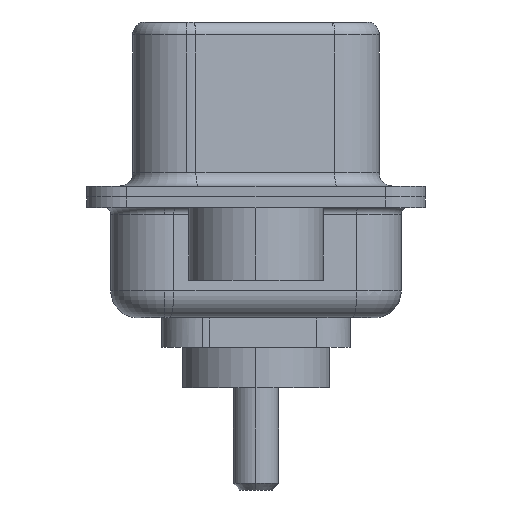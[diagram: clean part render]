
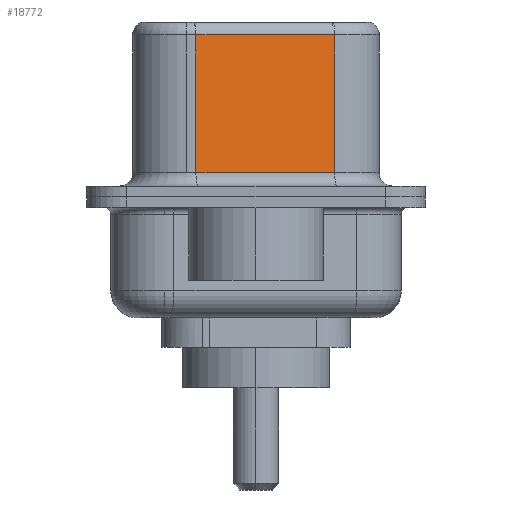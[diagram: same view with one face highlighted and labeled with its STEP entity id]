
A CAD part, left-side view. The second image highlights one B-rep face of the part: STEP entity #18772.
In plain terms, the highlighted planar face has unit normal (-0.985, -0.174, 0).
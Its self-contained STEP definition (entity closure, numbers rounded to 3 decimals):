
#377 = EDGE_LOOP ( 'NONE', ( #16490, #16355, #4769, #13958 ) ) ;
#455 = EDGE_CURVE ( 'NONE', #14845, #7604, #10488, .T. ) ;
#514 = EDGE_CURVE ( 'NONE', #8556, #4223, #520, .T. ) ;
#520 = LINE ( 'NONE', #18550, #5027 ) ;
#2839 = LINE ( 'NONE', #10534, #11919 ) ;
#3498 = DIRECTION ( 'NONE',  ( -0.174, 0.985, 0. ) ) ;
#3651 = CARTESIAN_POINT ( 'NONE',  ( 3.67, 2.233, 6.52 ) ) ;
#3732 = DIRECTION ( 'NONE',  ( 0.985, 0.174, 0. ) ) ;
#4147 = LINE ( 'NONE', #3651, #4860 ) ;
#4223 = VERTEX_POINT ( 'NONE', #9296 ) ;
#4769 = ORIENTED_EDGE ( 'NONE', *, *, #16687, .T. ) ;
#4860 = VECTOR ( 'NONE', #18268, 1000. ) ;
#5027 = VECTOR ( 'NONE', #13930, 1000. ) ;
#5991 = CARTESIAN_POINT ( 'NONE',  ( 4.58, -2.927, 6.02 ) ) ;
#7093 = DIRECTION ( 'NONE',  ( -0.174, 0.985, 0. ) ) ;
#7278 = CARTESIAN_POINT ( 'NONE',  ( 3.67, 2.233, 0.9 ) ) ;
#7604 = VERTEX_POINT ( 'NONE', #16221 ) ;
#8195 = PLANE ( 'NONE',  #8287 ) ;
#8287 = AXIS2_PLACEMENT_3D ( 'NONE', #18180, #3732, #7093 ) ;
#8556 = VERTEX_POINT ( 'NONE', #7278 ) ;
#9296 = CARTESIAN_POINT ( 'NONE',  ( 4.58, -2.927, 0.9 ) ) ;
#9544 = CARTESIAN_POINT ( 'NONE',  ( 4.58, -2.927, 6.02 ) ) ;
#10476 = DIRECTION ( 'NONE',  ( 0., 0., -1. ) ) ;
#10488 = LINE ( 'NONE', #9544, #17499 ) ;
#10534 = CARTESIAN_POINT ( 'NONE',  ( 4.58, -2.927, 6.52 ) ) ;
#11919 = VECTOR ( 'NONE', #10476, 1000. ) ;
#13930 = DIRECTION ( 'NONE',  ( 0.174, -0.985, 0. ) ) ;
#13958 = ORIENTED_EDGE ( 'NONE', *, *, #514, .T. ) ;
#14845 = VERTEX_POINT ( 'NONE', #5991 ) ;
#15698 = EDGE_CURVE ( 'NONE', #14845, #4223, #2839, .T. ) ;
#16221 = CARTESIAN_POINT ( 'NONE',  ( 3.67, 2.233, 6.02 ) ) ;
#16355 = ORIENTED_EDGE ( 'NONE', *, *, #455, .T. ) ;
#16490 = ORIENTED_EDGE ( 'NONE', *, *, #15698, .F. ) ;
#16687 = EDGE_CURVE ( 'NONE', #7604, #8556, #4147, .T. ) ;
#17499 = VECTOR ( 'NONE', #3498, 1000. ) ;
#18164 = FACE_OUTER_BOUND ( 'NONE', #377, .T. ) ;
#18180 = CARTESIAN_POINT ( 'NONE',  ( 4.58, -2.927, 6.52 ) ) ;
#18268 = DIRECTION ( 'NONE',  ( 0., 0., -1. ) ) ;
#18550 = CARTESIAN_POINT ( 'NONE',  ( 4.58, -2.927, 0.9 ) ) ;
#18772 = ADVANCED_FACE ( 'NONE', ( #18164 ), #8195, .F. ) ;
